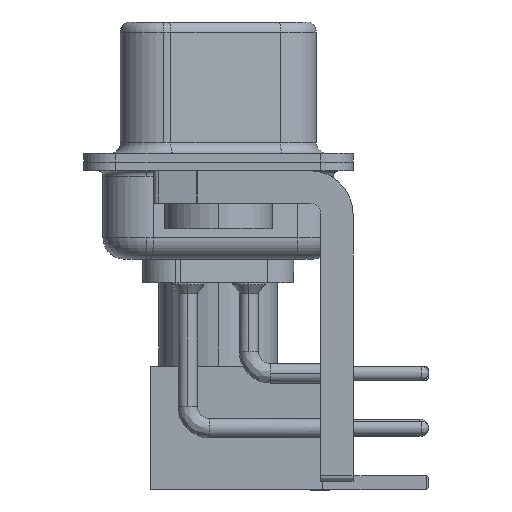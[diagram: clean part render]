
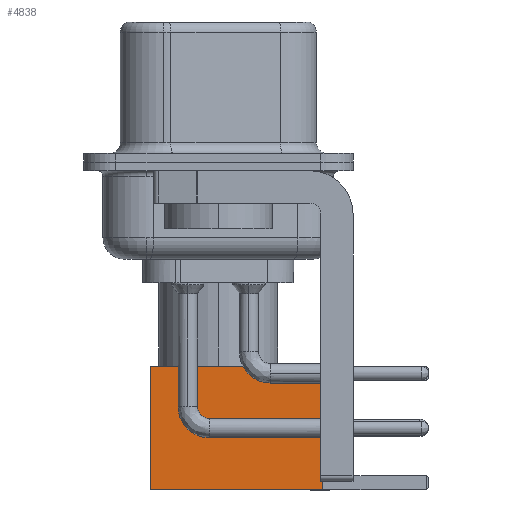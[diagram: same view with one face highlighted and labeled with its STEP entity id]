
A CAD part, left-side view. The second image highlights one B-rep face of the part: STEP entity #4838.
In plain terms, the highlighted face is planar.
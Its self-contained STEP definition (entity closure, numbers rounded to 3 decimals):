
#970 = ORIENTED_EDGE ( 'NONE', *, *, #21291, .F. ) ;
#2231 = CARTESIAN_POINT ( 'NONE',  ( 2.875, 2.875, 0. ) ) ;
#2383 = CARTESIAN_POINT ( 'NONE',  ( 2.875, 2.875, 0. ) ) ;
#3106 = EDGE_CURVE ( 'NONE', #17566, #22710, #13875, .T. ) ;
#3251 = VERTEX_POINT ( 'NONE', #5130 ) ;
#3796 = CARTESIAN_POINT ( 'NONE',  ( 2.875, 2.875, 8. ) ) ;
#3942 = CARTESIAN_POINT ( 'NONE',  ( -2.875, 2.875, 0. ) ) ;
#4838 = ADVANCED_FACE ( 'NONE', ( #22721 ), #12955, .T. ) ;
#5130 = CARTESIAN_POINT ( 'NONE',  ( 2.875, 2.875, 0. ) ) ;
#7243 = VECTOR ( 'NONE', #13823, 1000. ) ;
#7615 = ORIENTED_EDGE ( 'NONE', *, *, #3106, .F. ) ;
#8009 = DIRECTION ( 'NONE',  ( 0., 0., 1. ) ) ;
#8459 = VECTOR ( 'NONE', #16956, 1000. ) ;
#8484 = CARTESIAN_POINT ( 'NONE',  ( 0., 2.875, 8. ) ) ;
#8678 = CARTESIAN_POINT ( 'NONE',  ( 0., 2.875, 0. ) ) ;
#9257 = ORIENTED_EDGE ( 'NONE', *, *, #15286, .T. ) ;
#9638 = EDGE_CURVE ( 'NONE', #3251, #9868, #21539, .T. ) ;
#9868 = VERTEX_POINT ( 'NONE', #12595 ) ;
#9968 = DIRECTION ( 'NONE',  ( -1., 0., 0. ) ) ;
#11355 = VECTOR ( 'NONE', #9968, 1000. ) ;
#12595 = CARTESIAN_POINT ( 'NONE',  ( -2.875, 2.875, 0. ) ) ;
#12955 = PLANE ( 'NONE',  #17302 ) ;
#13413 = LINE ( 'NONE', #3942, #8459 ) ;
#13823 = DIRECTION ( 'NONE',  ( -1., 0., 0. ) ) ;
#13875 = LINE ( 'NONE', #8484, #11355 ) ;
#14647 = CARTESIAN_POINT ( 'NONE',  ( -2.875, 2.875, 8. ) ) ;
#15286 = EDGE_CURVE ( 'NONE', #17566, #3251, #22989, .T. ) ;
#15975 = ORIENTED_EDGE ( 'NONE', *, *, #9638, .T. ) ;
#16878 = VECTOR ( 'NONE', #18824, 1000. ) ;
#16956 = DIRECTION ( 'NONE',  ( 0., 0., -1. ) ) ;
#17302 = AXIS2_PLACEMENT_3D ( 'NONE', #2231, #20876, #8009 ) ;
#17566 = VERTEX_POINT ( 'NONE', #3796 ) ;
#18824 = DIRECTION ( 'NONE',  ( 0., 0., -1. ) ) ;
#20876 = DIRECTION ( 'NONE',  ( 0., 1., 0. ) ) ;
#21291 = EDGE_CURVE ( 'NONE', #22710, #9868, #13413, .T. ) ;
#21539 = LINE ( 'NONE', #8678, #7243 ) ;
#22710 = VERTEX_POINT ( 'NONE', #14647 ) ;
#22721 = FACE_OUTER_BOUND ( 'NONE', #22870, .T. ) ;
#22870 = EDGE_LOOP ( 'NONE', ( #9257, #15975, #970, #7615 ) ) ;
#22989 = LINE ( 'NONE', #2383, #16878 ) ;
